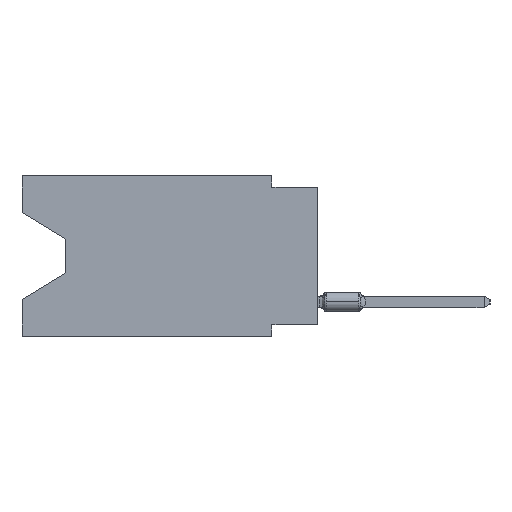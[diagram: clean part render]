
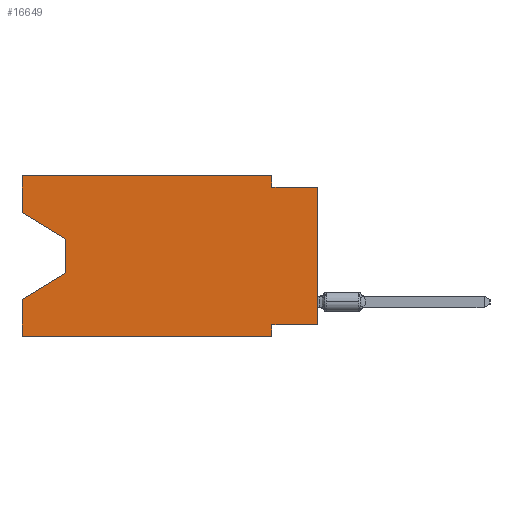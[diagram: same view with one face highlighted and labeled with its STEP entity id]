
A CAD part, left-side view. The second image highlights one B-rep face of the part: STEP entity #16649.
In plain terms, the highlighted planar face has unit normal (-1, 0, 0).
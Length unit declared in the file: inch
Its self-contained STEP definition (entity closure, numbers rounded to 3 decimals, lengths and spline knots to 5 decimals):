
#66 = CARTESIAN_POINT ( 'NONE',  ( 0., 0.645, 0. ) ) ;
#92 = CARTESIAN_POINT ( 'NONE',  ( 0., 0.1, -0.325 ) ) ;
#187 = VECTOR ( 'NONE', #16185, 39.37008 ) ;
#831 = CARTESIAN_POINT ( 'NONE',  ( 0., 0.645, -0.08025 ) ) ;
#1010 = VECTOR ( 'NONE', #25834, 39.37008 ) ;
#1207 = EDGE_CURVE ( 'NONE', #17508, #24353, #6717, .T. ) ;
#1367 = CARTESIAN_POINT ( 'NONE',  ( 0., 0.1, -0.025 ) ) ;
#1506 = LINE ( 'NONE', #25423, #12182 ) ;
#1957 = EDGE_CURVE ( 'NONE', #11371, #5890, #8230, .T. ) ;
#2078 = DIRECTION ( 'NONE',  ( 0., -0.855, -0.519 ) ) ;
#2494 = VERTEX_POINT ( 'NONE', #17166 ) ;
#2796 = DIRECTION ( 'NONE',  ( 0., 0., -1. ) ) ;
#3051 = VERTEX_POINT ( 'NONE', #21847 ) ;
#3393 = VECTOR ( 'NONE', #19273, 39.37008 ) ;
#3585 = VECTOR ( 'NONE', #21221, 39.37008 ) ;
#3630 = LINE ( 'NONE', #17468, #10666 ) ;
#4086 = PLANE ( 'NONE',  #25593 ) ;
#4132 = VERTEX_POINT ( 'NONE', #11002 ) ;
#4203 = FACE_OUTER_BOUND ( 'NONE', #4959, .T. ) ;
#4545 = VECTOR ( 'NONE', #11459, 39.37008 ) ;
#4558 = LINE ( 'NONE', #16821, #5582 ) ;
#4689 = DIRECTION ( 'NONE',  ( 0., -1., 0. ) ) ;
#4708 = VERTEX_POINT ( 'NONE', #92 ) ;
#4959 = EDGE_LOOP ( 'NONE', ( #25290, #6236, #22637, #20877, #15945, #22671, #21824, #8902, #17425, #13810, #22389, #8937 ) ) ;
#5565 = CARTESIAN_POINT ( 'NONE',  ( 0., 0., -0.325 ) ) ;
#5582 = VECTOR ( 'NONE', #4689, 39.37008 ) ;
#5781 = CARTESIAN_POINT ( 'NONE',  ( 0., 0., 0. ) ) ;
#5850 = CARTESIAN_POINT ( 'NONE',  ( 0., 0.645, 0. ) ) ;
#5890 = VERTEX_POINT ( 'NONE', #15658 ) ;
#6173 = DIRECTION ( 'NONE',  ( 1., 0., 0. ) ) ;
#6236 = ORIENTED_EDGE ( 'NONE', *, *, #1957, .T. ) ;
#6618 = CARTESIAN_POINT ( 'NONE',  ( 0., 0.1, -0.35 ) ) ;
#6717 = LINE ( 'NONE', #19012, #9270 ) ;
#6797 = CARTESIAN_POINT ( 'NONE',  ( 0., 0.55, -0.138 ) ) ;
#8219 = LINE ( 'NONE', #18258, #1010 ) ;
#8230 = LINE ( 'NONE', #20372, #187 ) ;
#8902 = ORIENTED_EDGE ( 'NONE', *, *, #14301, .T. ) ;
#8937 = ORIENTED_EDGE ( 'NONE', *, *, #13410, .F. ) ;
#9270 = VECTOR ( 'NONE', #2796, 39.37008 ) ;
#9455 = EDGE_CURVE ( 'NONE', #4132, #13593, #13259, .T. ) ;
#10017 = DIRECTION ( 'NONE',  ( 0., 0., 1. ) ) ;
#10018 = LINE ( 'NONE', #66, #18096 ) ;
#10270 = EDGE_CURVE ( 'NONE', #4708, #13593, #23494, .T. ) ;
#10666 = VECTOR ( 'NONE', #10017, 39.37008 ) ;
#11002 = CARTESIAN_POINT ( 'NONE',  ( 0., 0.645, -0.35 ) ) ;
#11371 = VERTEX_POINT ( 'NONE', #6797 ) ;
#11459 = DIRECTION ( 'NONE',  ( 0., 0., -1. ) ) ;
#11706 = VERTEX_POINT ( 'NONE', #831 ) ;
#11910 = EDGE_CURVE ( 'NONE', #5890, #2494, #1506, .T. ) ;
#12182 = VECTOR ( 'NONE', #15223, 39.37008 ) ;
#13259 = LINE ( 'NONE', #16921, #3393 ) ;
#13410 = EDGE_CURVE ( 'NONE', #11706, #25842, #3630, .T. ) ;
#13420 = CARTESIAN_POINT ( 'NONE',  ( 0., 0.1, -0.35 ) ) ;
#13537 = DIRECTION ( 'NONE',  ( 0., 1., 0. ) ) ;
#13593 = VERTEX_POINT ( 'NONE', #6618 ) ;
#13810 = ORIENTED_EDGE ( 'NONE', *, *, #1207, .F. ) ;
#14301 = EDGE_CURVE ( 'NONE', #3051, #19984, #23694, .T. ) ;
#14463 = CARTESIAN_POINT ( 'NONE',  ( 0., 0.1, 0. ) ) ;
#15127 = EDGE_CURVE ( 'NONE', #3051, #4708, #19549, .T. ) ;
#15223 = DIRECTION ( 'NONE',  ( 0., 0.855, -0.519 ) ) ;
#15658 = CARTESIAN_POINT ( 'NONE',  ( 0., 0.55, -0.212 ) ) ;
#15937 = LINE ( 'NONE', #16448, #19780 ) ;
#15945 = ORIENTED_EDGE ( 'NONE', *, *, #9455, .T. ) ;
#16185 = DIRECTION ( 'NONE',  ( 0., 0., -1. ) ) ;
#16448 = CARTESIAN_POINT ( 'NONE',  ( 0., 0.645, -0.08025 ) ) ;
#16649 = ADVANCED_FACE ( 'NONE', ( #4203 ), #4086, .F. ) ;
#16821 = CARTESIAN_POINT ( 'NONE',  ( 0., 0., -0.025 ) ) ;
#16921 = CARTESIAN_POINT ( 'NONE',  ( 0., 0.645, -0.35 ) ) ;
#17062 = CARTESIAN_POINT ( 'NONE',  ( 0., 0., -0.025 ) ) ;
#17158 = EDGE_CURVE ( 'NONE', #24353, #19984, #4558, .T. ) ;
#17166 = CARTESIAN_POINT ( 'NONE',  ( 0., 0.645, -0.26975 ) ) ;
#17425 = ORIENTED_EDGE ( 'NONE', *, *, #17158, .F. ) ;
#17468 = CARTESIAN_POINT ( 'NONE',  ( 0., 0.645, 0. ) ) ;
#17498 = EDGE_CURVE ( 'NONE', #25842, #17508, #10018, .T. ) ;
#17508 = VERTEX_POINT ( 'NONE', #14463 ) ;
#18096 = VECTOR ( 'NONE', #24147, 39.37008 ) ;
#18258 = CARTESIAN_POINT ( 'NONE',  ( 0., 0.645, 0. ) ) ;
#18668 = EDGE_CURVE ( 'NONE', #4132, #2494, #8219, .T. ) ;
#19012 = CARTESIAN_POINT ( 'NONE',  ( 0., 0.1, 0. ) ) ;
#19273 = DIRECTION ( 'NONE',  ( 0., -1., 0. ) ) ;
#19549 = LINE ( 'NONE', #5565, #20329 ) ;
#19780 = VECTOR ( 'NONE', #2078, 39.37008 ) ;
#19984 = VERTEX_POINT ( 'NONE', #17062 ) ;
#20329 = VECTOR ( 'NONE', #13537, 39.37008 ) ;
#20372 = CARTESIAN_POINT ( 'NONE',  ( 0., 0.55, -0.138 ) ) ;
#20877 = ORIENTED_EDGE ( 'NONE', *, *, #18668, .F. ) ;
#21221 = DIRECTION ( 'NONE',  ( 0., 0., 1. ) ) ;
#21824 = ORIENTED_EDGE ( 'NONE', *, *, #15127, .F. ) ;
#21847 = CARTESIAN_POINT ( 'NONE',  ( 0., 0., -0.325 ) ) ;
#22242 = CARTESIAN_POINT ( 'NONE',  ( 0., 0.645, 0. ) ) ;
#22389 = ORIENTED_EDGE ( 'NONE', *, *, #17498, .F. ) ;
#22637 = ORIENTED_EDGE ( 'NONE', *, *, #11910, .T. ) ;
#22671 = ORIENTED_EDGE ( 'NONE', *, *, #10270, .F. ) ;
#23494 = LINE ( 'NONE', #13420, #4545 ) ;
#23694 = LINE ( 'NONE', #5781, #3585 ) ;
#24147 = DIRECTION ( 'NONE',  ( 0., -1., 0. ) ) ;
#24329 = DIRECTION ( 'NONE',  ( 0., 0., -1. ) ) ;
#24353 = VERTEX_POINT ( 'NONE', #1367 ) ;
#25290 = ORIENTED_EDGE ( 'NONE', *, *, #25479, .T. ) ;
#25423 = CARTESIAN_POINT ( 'NONE',  ( 0., 0.55, -0.212 ) ) ;
#25479 = EDGE_CURVE ( 'NONE', #11706, #11371, #15937, .T. ) ;
#25593 = AXIS2_PLACEMENT_3D ( 'NONE', #22242, #6173, #24329 ) ;
#25834 = DIRECTION ( 'NONE',  ( 0., 0., 1. ) ) ;
#25842 = VERTEX_POINT ( 'NONE', #5850 ) ;
